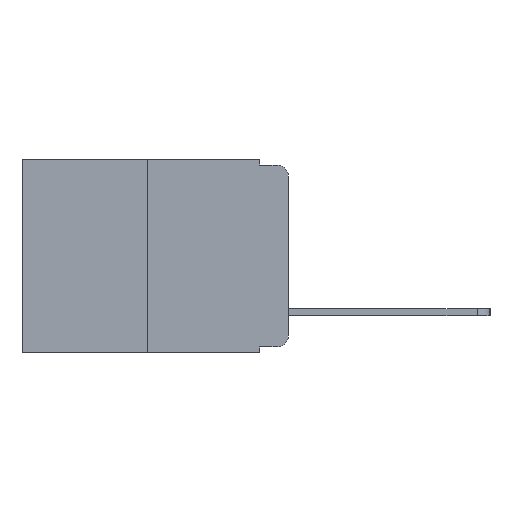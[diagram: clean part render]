
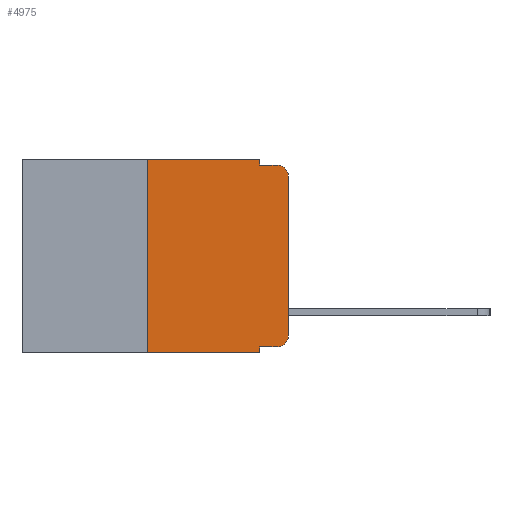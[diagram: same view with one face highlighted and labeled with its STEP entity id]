
A CAD part, left-side view. The second image highlights one B-rep face of the part: STEP entity #4975.
In plain terms, the highlighted planar face has unit normal (-1, 0, 0).
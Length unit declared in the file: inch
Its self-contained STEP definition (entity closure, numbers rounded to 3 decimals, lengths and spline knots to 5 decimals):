
#201 = DIRECTION ( 'NONE',  ( -1., 0., 0. ) ) ;
#744 = CARTESIAN_POINT ( 'NONE',  ( 0., 0.473, 0. ) ) ;
#819 = DIRECTION ( 'NONE',  ( 0., 0., 1. ) ) ;
#981 = CARTESIAN_POINT ( 'NONE',  ( 0., 0.473, -0.343 ) ) ;
#1099 = DIRECTION ( 'NONE',  ( 0., 0., -1. ) ) ;
#1204 = LINE ( 'NONE', #6450, #13422 ) ;
#1552 = VERTEX_POINT ( 'NONE', #14468 ) ;
#1624 = LINE ( 'NONE', #6703, #10488 ) ;
#2032 = AXIS2_PLACEMENT_3D ( 'NONE', #7250, #201, #8397 ) ;
#2259 = VECTOR ( 'NONE', #9134, 39.37008 ) ;
#2318 = VECTOR ( 'NONE', #3939, 39.37008 ) ;
#2679 = VECTOR ( 'NONE', #1099, 39.37008 ) ;
#2766 = CARTESIAN_POINT ( 'NONE',  ( 0., 0., 0. ) ) ;
#2854 = VECTOR ( 'NONE', #7623, 39.37008 ) ;
#3050 = LINE ( 'NONE', #13736, #8864 ) ;
#3125 = DIRECTION ( 'NONE',  ( 0., 0., -1. ) ) ;
#3142 = ORIENTED_EDGE ( 'NONE', *, *, #12334, .F. ) ;
#3208 = LINE ( 'NONE', #6464, #2854 ) ;
#3429 = CARTESIAN_POINT ( 'NONE',  ( 0., 0., -0.313 ) ) ;
#3445 = ORIENTED_EDGE ( 'NONE', *, *, #3927, .F. ) ;
#3638 = ORIENTED_EDGE ( 'NONE', *, *, #12537, .T. ) ;
#3738 = EDGE_CURVE ( 'NONE', #12488, #11502, #1624, .T. ) ;
#3912 = CARTESIAN_POINT ( 'NONE',  ( 0., 0.02, -0.333 ) ) ;
#3925 = CARTESIAN_POINT ( 'NONE',  ( 0., 0.02, -0.03 ) ) ;
#3927 = EDGE_CURVE ( 'NONE', #6405, #12286, #8380, .T. ) ;
#3939 = DIRECTION ( 'NONE',  ( 0., 0., 1. ) ) ;
#4212 = VERTEX_POINT ( 'NONE', #12021 ) ;
#4975 = ADVANCED_FACE ( 'NONE', ( #13812 ), #8907, .F. ) ;
#5103 = DIRECTION ( 'NONE',  ( 0., 0., -1. ) ) ;
#5344 = ORIENTED_EDGE ( 'NONE', *, *, #13673, .T. ) ;
#5398 = CARTESIAN_POINT ( 'NONE',  ( 0., 0.051, -0.01 ) ) ;
#5579 = ORIENTED_EDGE ( 'NONE', *, *, #11719, .F. ) ;
#5705 = DIRECTION ( 'NONE',  ( 0., -1., 0. ) ) ;
#5795 = CARTESIAN_POINT ( 'NONE',  ( 0., 0.051, 0. ) ) ;
#5804 = EDGE_CURVE ( 'NONE', #11320, #13248, #14865, .T. ) ;
#5805 = LINE ( 'NONE', #5795, #2679 ) ;
#6405 = VERTEX_POINT ( 'NONE', #13871 ) ;
#6450 = CARTESIAN_POINT ( 'NONE',  ( 0., 0.051, -0.333 ) ) ;
#6464 = CARTESIAN_POINT ( 'NONE',  ( 0., 0.051, 0. ) ) ;
#6703 = CARTESIAN_POINT ( 'NONE',  ( 0., 0.25, 0. ) ) ;
#6971 = VERTEX_POINT ( 'NONE', #13750 ) ;
#7190 = AXIS2_PLACEMENT_3D ( 'NONE', #744, #10024, #3125 ) ;
#7250 = CARTESIAN_POINT ( 'NONE',  ( 0., 0.02, -0.313 ) ) ;
#7623 = DIRECTION ( 'NONE',  ( 0., 0., -1. ) ) ;
#7729 = CARTESIAN_POINT ( 'NONE',  ( 0., 0.25, 0. ) ) ;
#7997 = ORIENTED_EDGE ( 'NONE', *, *, #11981, .T. ) ;
#8380 = LINE ( 'NONE', #5398, #11018 ) ;
#8397 = DIRECTION ( 'NONE',  ( 0., 0., -1. ) ) ;
#8466 = LINE ( 'NONE', #981, #2259 ) ;
#8527 = LINE ( 'NONE', #2766, #2318 ) ;
#8608 = ORIENTED_EDGE ( 'NONE', *, *, #12082, .T. ) ;
#8864 = VECTOR ( 'NONE', #14899, 39.37008 ) ;
#8907 = PLANE ( 'NONE',  #7190 ) ;
#9128 = CARTESIAN_POINT ( 'NONE',  ( 0., 0.02, -0.01 ) ) ;
#9134 = DIRECTION ( 'NONE',  ( 0., -1., 0. ) ) ;
#9803 = ORIENTED_EDGE ( 'NONE', *, *, #3738, .F. ) ;
#10024 = DIRECTION ( 'NONE',  ( 1., 0., 0. ) ) ;
#10067 = VERTEX_POINT ( 'NONE', #11710 ) ;
#10315 = EDGE_LOOP ( 'NONE', ( #7997, #3638, #3445, #11897, #3142, #9803, #5344, #5579, #8608, #12061 ) ) ;
#10488 = VECTOR ( 'NONE', #819, 39.37008 ) ;
#11018 = VECTOR ( 'NONE', #5705, 39.37008 ) ;
#11320 = VERTEX_POINT ( 'NONE', #3912 ) ;
#11502 = VERTEX_POINT ( 'NONE', #7729 ) ;
#11710 = CARTESIAN_POINT ( 'NONE',  ( 0., 0., -0.03 ) ) ;
#11719 = EDGE_CURVE ( 'NONE', #6971, #4212, #5805, .T. ) ;
#11897 = ORIENTED_EDGE ( 'NONE', *, *, #13009, .F. ) ;
#11940 = DIRECTION ( 'NONE',  ( -1., 0., 0. ) ) ;
#11981 = EDGE_CURVE ( 'NONE', #13248, #10067, #8527, .T. ) ;
#12021 = CARTESIAN_POINT ( 'NONE',  ( 0., 0.051, -0.343 ) ) ;
#12061 = ORIENTED_EDGE ( 'NONE', *, *, #5804, .T. ) ;
#12082 = EDGE_CURVE ( 'NONE', #6971, #11320, #1204, .T. ) ;
#12286 = VERTEX_POINT ( 'NONE', #9128 ) ;
#12334 = EDGE_CURVE ( 'NONE', #11502, #1552, #3050, .T. ) ;
#12488 = VERTEX_POINT ( 'NONE', #13987 ) ;
#12537 = EDGE_CURVE ( 'NONE', #10067, #12286, #13059, .T. ) ;
#13009 = EDGE_CURVE ( 'NONE', #1552, #6405, #3208, .T. ) ;
#13059 = CIRCLE ( 'NONE', #14113, 0.02 ) ;
#13196 = DIRECTION ( 'NONE',  ( 0., -1., 0. ) ) ;
#13248 = VERTEX_POINT ( 'NONE', #3429 ) ;
#13422 = VECTOR ( 'NONE', #13196, 39.37008 ) ;
#13673 = EDGE_CURVE ( 'NONE', #12488, #4212, #8466, .T. ) ;
#13736 = CARTESIAN_POINT ( 'NONE',  ( 0., 0.473, 0. ) ) ;
#13750 = CARTESIAN_POINT ( 'NONE',  ( 0., 0.051, -0.333 ) ) ;
#13812 = FACE_OUTER_BOUND ( 'NONE', #10315, .T. ) ;
#13871 = CARTESIAN_POINT ( 'NONE',  ( 0., 0.051, -0.01 ) ) ;
#13987 = CARTESIAN_POINT ( 'NONE',  ( 0., 0.25, -0.343 ) ) ;
#14113 = AXIS2_PLACEMENT_3D ( 'NONE', #3925, #11940, #5103 ) ;
#14468 = CARTESIAN_POINT ( 'NONE',  ( 0., 0.051, 0. ) ) ;
#14865 = CIRCLE ( 'NONE', #2032, 0.02 ) ;
#14899 = DIRECTION ( 'NONE',  ( 0., -1., 0. ) ) ;
